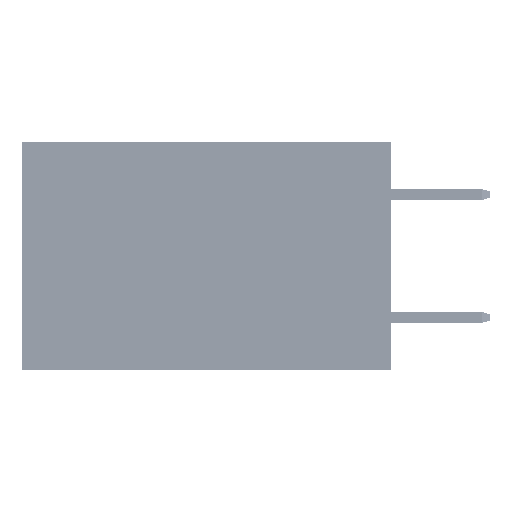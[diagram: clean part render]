
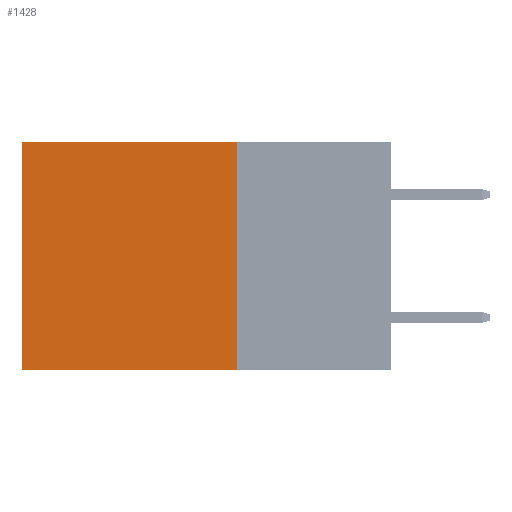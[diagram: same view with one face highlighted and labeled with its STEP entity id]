
A CAD part, left-side view. The second image highlights one B-rep face of the part: STEP entity #1428.
In plain terms, the highlighted planar face has unit normal (-1, 0, 0).
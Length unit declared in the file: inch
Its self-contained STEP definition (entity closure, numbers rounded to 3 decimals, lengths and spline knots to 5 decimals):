
#1428 = ADVANCED_FACE ( 'NONE', ( #27149 ), #7262, .F. ) ;
#2065 = VERTEX_POINT ( 'NONE', #44536 ) ;
#4114 = VERTEX_POINT ( 'NONE', #26725 ) ;
#5548 = LINE ( 'NONE', #49755, #13577 ) ;
#6451 = ORIENTED_EDGE ( 'NONE', *, *, #9282, .F. ) ;
#7262 = PLANE ( 'NONE',  #14522 ) ;
#7781 = DIRECTION ( 'NONE',  ( 0., 0., -1. ) ) ;
#7894 = DIRECTION ( 'NONE',  ( 0., 1., 0. ) ) ;
#8115 = EDGE_CURVE ( 'NONE', #2065, #15733, #11489, .T. ) ;
#9282 = EDGE_CURVE ( 'NONE', #15733, #4114, #11073, .T. ) ;
#10710 = CARTESIAN_POINT ( 'NONE',  ( 0.2875, 0.25, 0. ) ) ;
#10955 = DIRECTION ( 'NONE',  ( 1., 0., 0. ) ) ;
#10978 = VECTOR ( 'NONE', #7894, 39.37008 ) ;
#11073 = LINE ( 'NONE', #48401, #10978 ) ;
#11324 = EDGE_LOOP ( 'NONE', ( #39071, #6451, #17139, #20134 ) ) ;
#11489 = LINE ( 'NONE', #10710, #49363 ) ;
#13577 = VECTOR ( 'NONE', #41576, 39.37008 ) ;
#14522 = AXIS2_PLACEMENT_3D ( 'NONE', #42774, #10955, #14701 ) ;
#14701 = DIRECTION ( 'NONE',  ( 0., 0., -1. ) ) ;
#14768 = EDGE_CURVE ( 'NONE', #2065, #19823, #5548, .T. ) ;
#15733 = VERTEX_POINT ( 'NONE', #18134 ) ;
#17139 = ORIENTED_EDGE ( 'NONE', *, *, #8115, .F. ) ;
#18134 = CARTESIAN_POINT ( 'NONE',  ( 0.2875, 0.25, -0.37 ) ) ;
#18547 = LINE ( 'NONE', #46890, #35574 ) ;
#19823 = VERTEX_POINT ( 'NONE', #37287 ) ;
#20134 = ORIENTED_EDGE ( 'NONE', *, *, #14768, .T. ) ;
#26725 = CARTESIAN_POINT ( 'NONE',  ( 0.2875, 0.6, -0.37 ) ) ;
#27149 = FACE_OUTER_BOUND ( 'NONE', #11324, .T. ) ;
#35574 = VECTOR ( 'NONE', #39224, 39.37008 ) ;
#37287 = CARTESIAN_POINT ( 'NONE',  ( 0.2875, 0.6, 0. ) ) ;
#39071 = ORIENTED_EDGE ( 'NONE', *, *, #50267, .T. ) ;
#39224 = DIRECTION ( 'NONE',  ( 0., 0., -1. ) ) ;
#41576 = DIRECTION ( 'NONE',  ( 0., 1., 0. ) ) ;
#42774 = CARTESIAN_POINT ( 'NONE',  ( 0.2875, 0.25, 0. ) ) ;
#44536 = CARTESIAN_POINT ( 'NONE',  ( 0.2875, 0.25, 0. ) ) ;
#46890 = CARTESIAN_POINT ( 'NONE',  ( 0.2875, 0.6, 0. ) ) ;
#48401 = CARTESIAN_POINT ( 'NONE',  ( 0.2875, 0.25, -0.37 ) ) ;
#49363 = VECTOR ( 'NONE', #7781, 39.37008 ) ;
#49755 = CARTESIAN_POINT ( 'NONE',  ( 0.2875, 0.25, 0. ) ) ;
#50267 = EDGE_CURVE ( 'NONE', #19823, #4114, #18547, .T. ) ;
